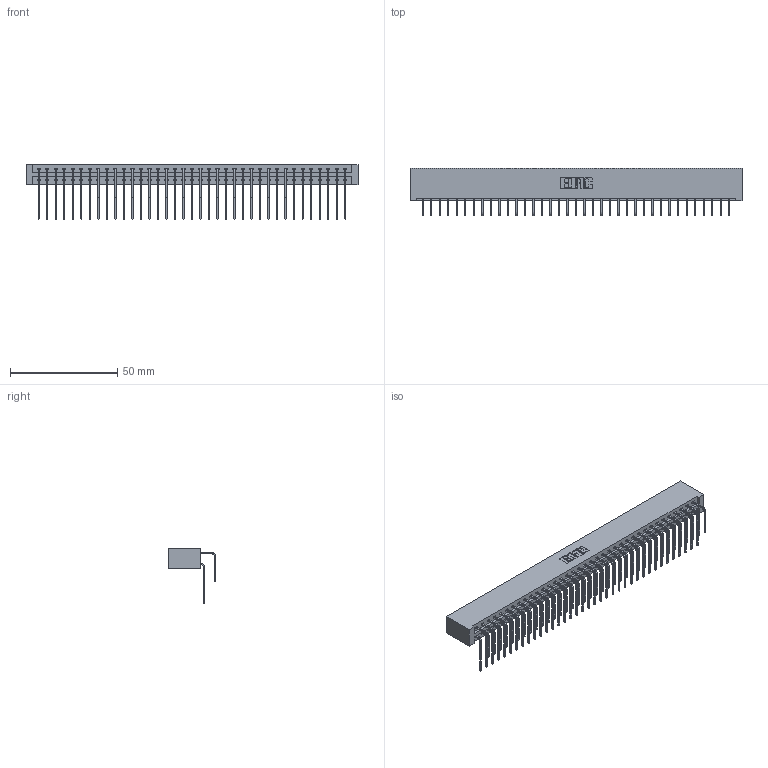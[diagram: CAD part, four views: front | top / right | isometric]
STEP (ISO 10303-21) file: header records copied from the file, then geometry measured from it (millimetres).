
FILE_DESCRIPTION (( 'STEP AP203' ), '1' );
FILE_NAME ('337-074-558-201.STEP', '2019-10-10T04:15:16', ( '' ), ( '' ), 'SwSTEP 2.0', 'SolidWorks 2016', '' );
FILE_SCHEMA (( 'CONFIG_CONTROL_DESIGN' ));
Length unit declared in the file: inch
Products named in the file (4): 345-292-001_558 559 Tail - 1; 337 Part_No Mounting Lugs; 337-074-558-201; 345-292-001_558 Tail - 2
Assembly tree (75 placements, depth 2):
  337-074-558-201
    337 Part_No Mounting Lugs
    345-292-001_558 559 Tail - 1  x37
    345-292-001_558 Tail - 2  x37
Bounding box: 154.48 x 22.17 x 25.53 mm (x, y, z)
Volume: 17401.7 mm3; surface area: 21823.7 mm2
Topology: 75 solids, 75 shells, 4250 faces, 12645 edges, 8330 vertices
Faces by surface type: plane 3026, cylinder 1224
Entity records: 30841 total; most frequent: CARTESIAN_POINT 5245, ORIENTED_EDGE 5130, DIRECTION 4445, EDGE_CURVE 2565, VECTOR 2405, LINE 2405, VERTEX_POINT 1706, AXIS2_PLACEMENT_3D 1020
